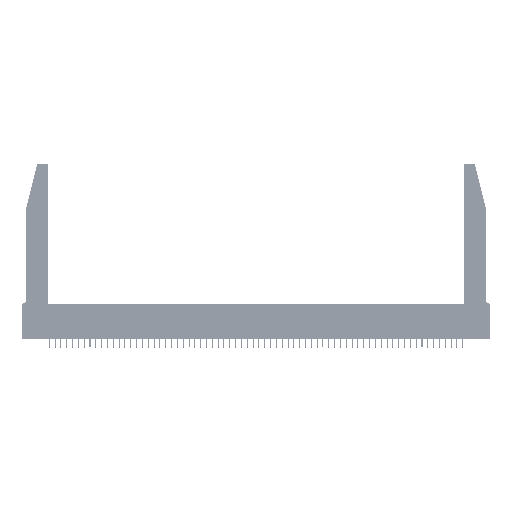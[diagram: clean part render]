
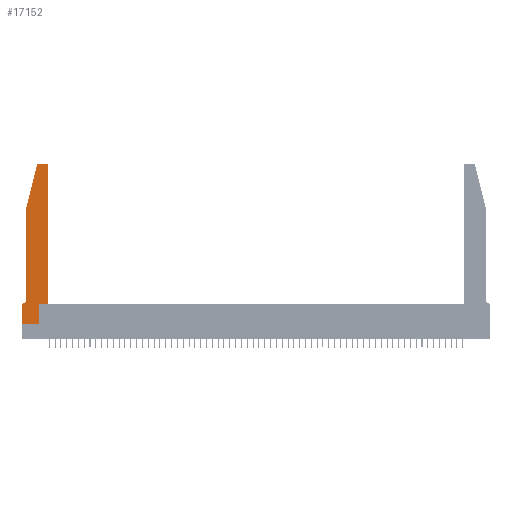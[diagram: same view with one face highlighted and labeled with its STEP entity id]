
A CAD part, top view. The second image highlights one B-rep face of the part: STEP entity #17152.
In plain terms, the highlighted planar face has unit normal (0, 0, 1).
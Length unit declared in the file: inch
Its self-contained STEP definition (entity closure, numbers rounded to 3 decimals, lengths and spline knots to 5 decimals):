
#1067 = DIRECTION ( 'NONE',  ( 1., 0., 0. ) ) ;
#1882 = CARTESIAN_POINT ( 'NONE',  ( 0.0755, 2., 0.37 ) ) ;
#2221 = ORIENTED_EDGE ( 'NONE', *, *, #41538, .T. ) ;
#3566 = CARTESIAN_POINT ( 'NONE',  ( 0., 0.35, 0.37 ) ) ;
#4958 = CARTESIAN_POINT ( 'NONE',  ( 0.4205, 2.75, 0.37 ) ) ;
#5790 = VERTEX_POINT ( 'NONE', #45234 ) ;
#6532 = DIRECTION ( 'NONE',  ( -1., 0., 0. ) ) ;
#6931 = VERTEX_POINT ( 'NONE', #4958 ) ;
#7285 = ORIENTED_EDGE ( 'NONE', *, *, #36399, .T. ) ;
#7802 = ORIENTED_EDGE ( 'NONE', *, *, #41567, .T. ) ;
#8483 = FACE_OUTER_BOUND ( 'NONE', #31548, .T. ) ;
#8736 = LINE ( 'NONE', #31877, #54326 ) ;
#9424 = EDGE_CURVE ( 'NONE', #50509, #21255, #8736, .T. ) ;
#9449 = LINE ( 'NONE', #41578, #44740 ) ;
#10467 = EDGE_CURVE ( 'NONE', #37419, #20496, #47352, .T. ) ;
#10761 = CARTESIAN_POINT ( 'NONE',  ( 0.25487, 2.72718, 0.37 ) ) ;
#10866 = CARTESIAN_POINT ( 'NONE',  ( 0.2605, 2.75, 0.37 ) ) ;
#11063 = CIRCLE ( 'NONE', #32512, 0.03 ) ;
#11605 = CARTESIAN_POINT ( 'NONE',  ( 0.4205, 2.72, 0.37 ) ) ;
#11801 = VERTEX_POINT ( 'NONE', #10761 ) ;
#12163 = AXIS2_PLACEMENT_3D ( 'NONE', #15759, #46643, #20230 ) ;
#12859 = CARTESIAN_POINT ( 'NONE',  ( 0., 0.35, 0.37 ) ) ;
#13055 = DIRECTION ( 'NONE',  ( 1., 0., 0. ) ) ;
#13918 = CARTESIAN_POINT ( 'NONE',  ( 0.0055, 0.35, 0.37 ) ) ;
#15393 = VERTEX_POINT ( 'NONE', #13918 ) ;
#15759 = CARTESIAN_POINT ( 'NONE',  ( 0.0055, 0.42, 0.37 ) ) ;
#16094 = DIRECTION ( 'NONE',  ( 1., 0., 0. ) ) ;
#17152 = ADVANCED_FACE ( 'NONE', ( #8483 ), #56934, .T. ) ;
#17618 = EDGE_CURVE ( 'NONE', #20496, #50509, #54790, .T. ) ;
#18290 = CIRCLE ( 'NONE', #12163, 0.07 ) ;
#18717 = DIRECTION ( 'NONE',  ( 0., 1., 0. ) ) ;
#19024 = VECTOR ( 'NONE', #48779, 39.37008 ) ;
#19648 = DIRECTION ( 'NONE',  ( -0.239, -0.971, 0. ) ) ;
#19955 = ORIENTED_EDGE ( 'NONE', *, *, #17618, .T. ) ;
#20230 = DIRECTION ( 'NONE',  ( -1., 0., 0. ) ) ;
#20276 = CARTESIAN_POINT ( 'NONE',  ( 0., 0., 0.37 ) ) ;
#20496 = VERTEX_POINT ( 'NONE', #51599 ) ;
#21255 = VERTEX_POINT ( 'NONE', #40766 ) ;
#21874 = LINE ( 'NONE', #50447, #43972 ) ;
#21910 = ORIENTED_EDGE ( 'NONE', *, *, #48192, .T. ) ;
#21949 = EDGE_CURVE ( 'NONE', #35503, #11801, #48052, .T. ) ;
#22136 = CARTESIAN_POINT ( 'NONE',  ( 0.2865, 0., 0.37 ) ) ;
#22360 = AXIS2_PLACEMENT_3D ( 'NONE', #12859, #39498, #13055 ) ;
#22399 = CARTESIAN_POINT ( 'NONE',  ( 0., 0., 0.37 ) ) ;
#24025 = DIRECTION ( 'NONE',  ( 0., -1., 0. ) ) ;
#24805 = CARTESIAN_POINT ( 'NONE',  ( 0.4505, 0.35, 0.37 ) ) ;
#26147 = ORIENTED_EDGE ( 'NONE', *, *, #9424, .T. ) ;
#27782 = DIRECTION ( 'NONE',  ( 0., 0., 1. ) ) ;
#27905 = VERTEX_POINT ( 'NONE', #3566 ) ;
#30484 = EDGE_CURVE ( 'NONE', #34937, #5790, #32708, .T. ) ;
#31294 = CARTESIAN_POINT ( 'NONE',  ( 0.284, 2.75, 0.37 ) ) ;
#31387 = VECTOR ( 'NONE', #37897, 39.37008 ) ;
#31548 = EDGE_LOOP ( 'NONE', ( #7802, #50712, #2221, #55591, #7285, #50233, #21910, #55092, #40730, #19955, #26147, #40042 ) ) ;
#31877 = CARTESIAN_POINT ( 'NONE',  ( 0.4505, 0.35, 0.37 ) ) ;
#32512 = AXIS2_PLACEMENT_3D ( 'NONE', #11605, #42535, #16094 ) ;
#32708 = LINE ( 'NONE', #1882, #41661 ) ;
#33588 = DIRECTION ( 'NONE',  ( -1., 0., 0. ) ) ;
#34937 = VERTEX_POINT ( 'NONE', #40615 ) ;
#35503 = VERTEX_POINT ( 'NONE', #31294 ) ;
#36117 = EDGE_CURVE ( 'NONE', #44541, #37419, #52751, .T. ) ;
#36399 = EDGE_CURVE ( 'NONE', #5790, #15393, #18290, .T. ) ;
#37419 = VERTEX_POINT ( 'NONE', #22136 ) ;
#37436 = DIRECTION ( 'NONE',  ( 0., -1., 0. ) ) ;
#37611 = AXIS2_PLACEMENT_3D ( 'NONE', #54126, #27782, #1067 ) ;
#37616 = CARTESIAN_POINT ( 'NONE',  ( 0.4505, 0.35, 0.37 ) ) ;
#37897 = DIRECTION ( 'NONE',  ( 1., 0., 0. ) ) ;
#39168 = VECTOR ( 'NONE', #33588, 39.37008 ) ;
#39498 = DIRECTION ( 'NONE',  ( 0., 0., 1. ) ) ;
#40042 = ORIENTED_EDGE ( 'NONE', *, *, #46360, .T. ) ;
#40615 = CARTESIAN_POINT ( 'NONE',  ( 0.0755, 2., 0.37 ) ) ;
#40730 = ORIENTED_EDGE ( 'NONE', *, *, #10467, .T. ) ;
#40766 = CARTESIAN_POINT ( 'NONE',  ( 0.4505, 2.72, 0.37 ) ) ;
#41194 = VECTOR ( 'NONE', #6532, 39.37008 ) ;
#41538 = EDGE_CURVE ( 'NONE', #11801, #34937, #21874, .T. ) ;
#41567 = EDGE_CURVE ( 'NONE', #6931, #35503, #52860, .T. ) ;
#41578 = CARTESIAN_POINT ( 'NONE',  ( 0., 0., 0.37 ) ) ;
#41661 = VECTOR ( 'NONE', #37436, 39.37008 ) ;
#42535 = DIRECTION ( 'NONE',  ( 0., 0., 1. ) ) ;
#43972 = VECTOR ( 'NONE', #19648, 39.37008 ) ;
#44541 = VERTEX_POINT ( 'NONE', #20276 ) ;
#44740 = VECTOR ( 'NONE', #24025, 39.37008 ) ;
#45122 = CARTESIAN_POINT ( 'NONE',  ( 0.2865, 0.35, 0.37 ) ) ;
#45184 = DIRECTION ( 'NONE',  ( 0., 1., 0. ) ) ;
#45234 = CARTESIAN_POINT ( 'NONE',  ( 0.0755, 0.42, 0.37 ) ) ;
#46360 = EDGE_CURVE ( 'NONE', #21255, #6931, #11063, .T. ) ;
#46643 = DIRECTION ( 'NONE',  ( 0., 0., -1. ) ) ;
#47352 = LINE ( 'NONE', #45122, #48724 ) ;
#48052 = CIRCLE ( 'NONE', #37611, 0.03 ) ;
#48192 = EDGE_CURVE ( 'NONE', #27905, #44541, #9449, .T. ) ;
#48724 = VECTOR ( 'NONE', #18717, 39.37008 ) ;
#48779 = DIRECTION ( 'NONE',  ( 1., 0., 0. ) ) ;
#50233 = ORIENTED_EDGE ( 'NONE', *, *, #54555, .T. ) ;
#50447 = CARTESIAN_POINT ( 'NONE',  ( 0.0755, 2., 0.37 ) ) ;
#50509 = VERTEX_POINT ( 'NONE', #37616 ) ;
#50712 = ORIENTED_EDGE ( 'NONE', *, *, #21949, .T. ) ;
#51599 = CARTESIAN_POINT ( 'NONE',  ( 0.2865, 0.35, 0.37 ) ) ;
#52247 = LINE ( 'NONE', #55473, #39168 ) ;
#52751 = LINE ( 'NONE', #22399, #19024 ) ;
#52860 = LINE ( 'NONE', #10866, #41194 ) ;
#54126 = CARTESIAN_POINT ( 'NONE',  ( 0.284, 2.72, 0.37 ) ) ;
#54326 = VECTOR ( 'NONE', #45184, 39.37008 ) ;
#54555 = EDGE_CURVE ( 'NONE', #15393, #27905, #52247, .T. ) ;
#54790 = LINE ( 'NONE', #24805, #31387 ) ;
#55092 = ORIENTED_EDGE ( 'NONE', *, *, #36117, .T. ) ;
#55473 = CARTESIAN_POINT ( 'NONE',  ( 0.0755, 0.35, 0.37 ) ) ;
#55591 = ORIENTED_EDGE ( 'NONE', *, *, #30484, .T. ) ;
#56934 = PLANE ( 'NONE',  #22360 ) ;
